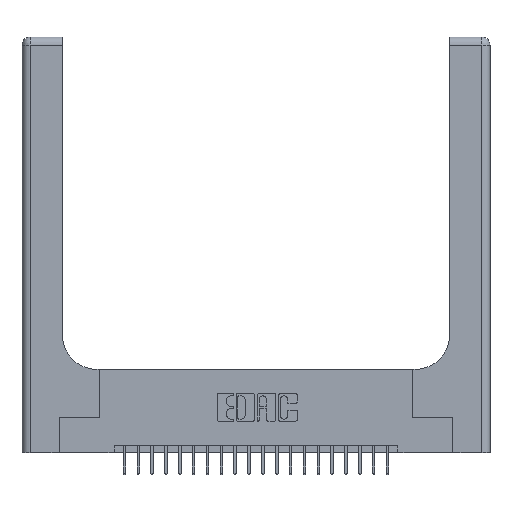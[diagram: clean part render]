
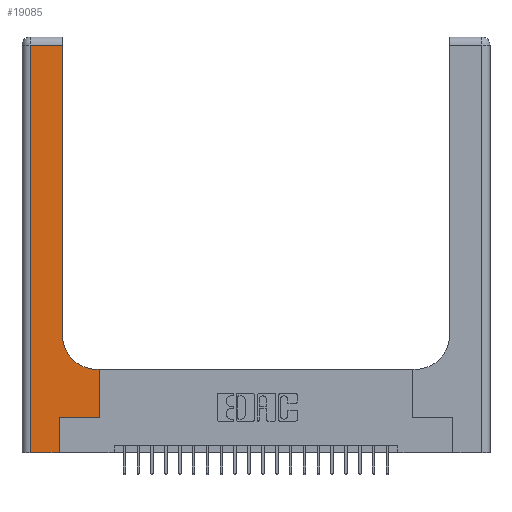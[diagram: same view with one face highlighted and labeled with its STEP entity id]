
A CAD part, top view. The second image highlights one B-rep face of the part: STEP entity #19085.
In plain terms, the highlighted planar face has unit normal (0, 0, 1).
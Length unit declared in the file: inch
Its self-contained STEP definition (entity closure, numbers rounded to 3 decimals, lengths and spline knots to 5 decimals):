
#887 = EDGE_CURVE ( 'NONE', #5075, #5762, #17455, .T. ) ;
#3056 = VECTOR ( 'NONE', #16346, 39.37008 ) ;
#3504 = CARTESIAN_POINT ( 'NONE',  ( 0.2915, 2.94, 0.37 ) ) ;
#3681 = CARTESIAN_POINT ( 'NONE',  ( 0.2915, 3., 0.37 ) ) ;
#3847 = VECTOR ( 'NONE', #19720, 39.37008 ) ;
#4035 = DIRECTION ( 'NONE',  ( 1., 0., 0. ) ) ;
#4065 = DIRECTION ( 'NONE',  ( 0., 1., 0. ) ) ;
#4162 = EDGE_CURVE ( 'NONE', #8572, #7471, #8176, .T. ) ;
#4267 = VECTOR ( 'NONE', #13193, 39.37008 ) ;
#4339 = LINE ( 'NONE', #3681, #23403 ) ;
#4832 = VERTEX_POINT ( 'NONE', #15806 ) ;
#5021 = EDGE_CURVE ( 'NONE', #6348, #12460, #11045, .T. ) ;
#5075 = VERTEX_POINT ( 'NONE', #3504 ) ;
#5544 = ORIENTED_EDGE ( 'NONE', *, *, #6978, .T. ) ;
#5656 = VECTOR ( 'NONE', #7257, 39.37008 ) ;
#5762 = VERTEX_POINT ( 'NONE', #9226 ) ;
#5914 = EDGE_CURVE ( 'NONE', #9305, #8572, #21330, .T. ) ;
#6348 = VERTEX_POINT ( 'NONE', #10824 ) ;
#6618 = VECTOR ( 'NONE', #4035, 39.37008 ) ;
#6978 = EDGE_CURVE ( 'NONE', #7471, #4832, #10366, .T. ) ;
#7257 = DIRECTION ( 'NONE',  ( 0., 1., 0. ) ) ;
#7449 = FACE_OUTER_BOUND ( 'NONE', #16762, .T. ) ;
#7471 = VERTEX_POINT ( 'NONE', #17808 ) ;
#7513 = EDGE_CURVE ( 'NONE', #4832, #15307, #11767, .T. ) ;
#7577 = CARTESIAN_POINT ( 'NONE',  ( 0., 3., 0.37 ) ) ;
#8031 = ORIENTED_EDGE ( 'NONE', *, *, #13550, .T. ) ;
#8051 = LINE ( 'NONE', #10838, #3056 ) ;
#8176 = LINE ( 'NONE', #22567, #13080 ) ;
#8572 = VERTEX_POINT ( 'NONE', #11389 ) ;
#9226 = CARTESIAN_POINT ( 'NONE',  ( 0.06, 2.94, 0.37 ) ) ;
#9275 = LINE ( 'NONE', #9508, #4267 ) ;
#9305 = VERTEX_POINT ( 'NONE', #11587 ) ;
#9447 = DIRECTION ( 'NONE',  ( 0., 0., -1. ) ) ;
#9508 = CARTESIAN_POINT ( 'NONE',  ( 0.2915, 0.6, 0.37 ) ) ;
#9798 = CARTESIAN_POINT ( 'NONE',  ( 0.2915, 0.85, 0.37 ) ) ;
#10366 = LINE ( 'NONE', #16293, #18980 ) ;
#10824 = CARTESIAN_POINT ( 'NONE',  ( 0.5415, 0.6, 0.37 ) ) ;
#10838 = CARTESIAN_POINT ( 'NONE',  ( 0.06, 3., 0.37 ) ) ;
#10872 = CARTESIAN_POINT ( 'NONE',  ( 0.5415, 0.85, 0.37 ) ) ;
#10890 = ORIENTED_EDGE ( 'NONE', *, *, #18483, .T. ) ;
#10925 = CARTESIAN_POINT ( 'NONE',  ( 0.5585, 0.25, 0.37 ) ) ;
#11045 = CIRCLE ( 'NONE', #14466, 0.25 ) ;
#11389 = CARTESIAN_POINT ( 'NONE',  ( 0.269, 0., 0.37 ) ) ;
#11473 = CARTESIAN_POINT ( 'NONE',  ( 0., 0., 0.37 ) ) ;
#11587 = CARTESIAN_POINT ( 'NONE',  ( 0.06, 0., 0.37 ) ) ;
#11767 = LINE ( 'NONE', #10925, #5656 ) ;
#12460 = VERTEX_POINT ( 'NONE', #9798 ) ;
#12710 = DIRECTION ( 'NONE',  ( 1., 0., 0. ) ) ;
#13080 = VECTOR ( 'NONE', #4065, 39.37008 ) ;
#13193 = DIRECTION ( 'NONE',  ( -1., 0., 0. ) ) ;
#13550 = EDGE_CURVE ( 'NONE', #15307, #6348, #9275, .T. ) ;
#14466 = AXIS2_PLACEMENT_3D ( 'NONE', #10872, #23686, #12710 ) ;
#14884 = PLANE ( 'NONE',  #21920 ) ;
#15212 = ORIENTED_EDGE ( 'NONE', *, *, #5914, .T. ) ;
#15307 = VERTEX_POINT ( 'NONE', #18176 ) ;
#15364 = EDGE_CURVE ( 'NONE', #12460, #5075, #4339, .T. ) ;
#15806 = CARTESIAN_POINT ( 'NONE',  ( 0.5585, 0.25, 0.37 ) ) ;
#16293 = CARTESIAN_POINT ( 'NONE',  ( 0.269, 0.25, 0.37 ) ) ;
#16346 = DIRECTION ( 'NONE',  ( 0., -1., 0. ) ) ;
#16762 = EDGE_LOOP ( 'NONE', ( #17231, #19585, #10890, #15212, #17933, #5544, #17354, #8031, #17476 ) ) ;
#17231 = ORIENTED_EDGE ( 'NONE', *, *, #15364, .T. ) ;
#17354 = ORIENTED_EDGE ( 'NONE', *, *, #7513, .T. ) ;
#17455 = LINE ( 'NONE', #19620, #3847 ) ;
#17476 = ORIENTED_EDGE ( 'NONE', *, *, #5021, .T. ) ;
#17808 = CARTESIAN_POINT ( 'NONE',  ( 0.269, 0.25, 0.37 ) ) ;
#17933 = ORIENTED_EDGE ( 'NONE', *, *, #4162, .T. ) ;
#18176 = CARTESIAN_POINT ( 'NONE',  ( 0.5585, 0.6, 0.37 ) ) ;
#18483 = EDGE_CURVE ( 'NONE', #5762, #9305, #8051, .T. ) ;
#18498 = DIRECTION ( 'NONE',  ( 0., 1., 0. ) ) ;
#18980 = VECTOR ( 'NONE', #20021, 39.37008 ) ;
#19085 = ADVANCED_FACE ( 'NONE', ( #7449 ), #14884, .F. ) ;
#19585 = ORIENTED_EDGE ( 'NONE', *, *, #887, .T. ) ;
#19620 = CARTESIAN_POINT ( 'NONE',  ( 0., 2.94, 0.37 ) ) ;
#19720 = DIRECTION ( 'NONE',  ( -1., 0., 0. ) ) ;
#20021 = DIRECTION ( 'NONE',  ( 1., 0., 0. ) ) ;
#21330 = LINE ( 'NONE', #11473, #6618 ) ;
#21920 = AXIS2_PLACEMENT_3D ( 'NONE', #7577, #9447, #22299 ) ;
#22299 = DIRECTION ( 'NONE',  ( -1., 0., 0. ) ) ;
#22567 = CARTESIAN_POINT ( 'NONE',  ( 0.269, 0., 0.37 ) ) ;
#23403 = VECTOR ( 'NONE', #18498, 39.37008 ) ;
#23686 = DIRECTION ( 'NONE',  ( 0., 0., -1. ) ) ;
